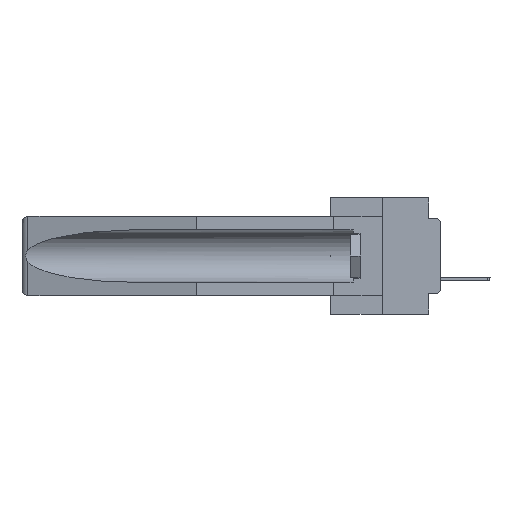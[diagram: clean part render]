
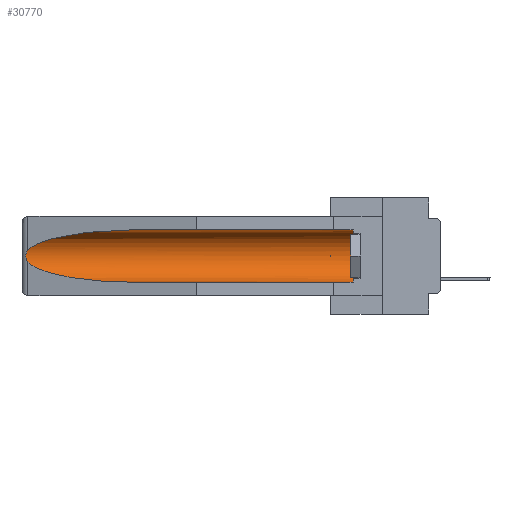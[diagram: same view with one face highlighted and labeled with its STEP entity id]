
A CAD part, left-side view. The second image highlights one B-rep face of the part: STEP entity #30770.
In plain terms, the highlighted cylindrical face has radius 2.857 mm (diameter 5.715 mm), a partial arc.
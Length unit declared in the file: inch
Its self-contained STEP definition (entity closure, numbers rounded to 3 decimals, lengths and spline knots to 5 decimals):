
#49 = CARTESIAN_POINT ( 'NONE',  ( 0.26537, 1.52718, -0.19328 ) ) ;
#94 = CARTESIAN_POINT ( 'NONE',  ( 0.155, 1.07973, -0.284 ) ) ;
#1596 = CARTESIAN_POINT ( 'NONE',  ( 0.26597, 1.52961, -0.15275 ) ) ;
#1840 = EDGE_LOOP ( 'NONE', ( #20788, #6467, #7239, #36404, #6667, #8755 ) ) ;
#1914 = CARTESIAN_POINT ( 'NONE',  ( 0.155, 0.126, -0.059 ) ) ;
#1947 =( BOUNDED_CURVE ( )  B_SPLINE_CURVE ( 3, ( #23305, #28876, #14259, #11176 ),
 .UNSPECIFIED., .F., .F. ) 
 B_SPLINE_CURVE_WITH_KNOTS ( ( 4, 4 ),
 ( 4.71239, 6.08839 ),
 .UNSPECIFIED. ) 
 CURVE ( )  GEOMETRIC_REPRESENTATION_ITEM ( )  RATIONAL_B_SPLINE_CURVE ( ( 1., 0.848, 0.848, 1. ) ) 
 REPRESENTATION_ITEM ( '' )  );
#1971 = EDGE_CURVE ( 'NONE', #37057, #34717, #27311, .T. ) ;
#2161 = AXIS2_PLACEMENT_3D ( 'NONE', #34331, #30947, #29024 ) ;
#4720 = CARTESIAN_POINT ( 'NONE',  ( 0.2675, 1.53308, -0.17534 ) ) ;
#4996 = CARTESIAN_POINT ( 'NONE',  ( 0.26537, 1.52718, -0.14972 ) ) ;
#5234 = CARTESIAN_POINT ( 'NONE',  ( 0.155, -0.30754, -0.1715 ) ) ;
#6221 = EDGE_CURVE ( 'NONE', #34717, #8247, #20496, .T. ) ;
#6467 = ORIENTED_EDGE ( 'NONE', *, *, #1971, .T. ) ;
#6667 = ORIENTED_EDGE ( 'NONE', *, *, #18655, .T. ) ;
#7239 = ORIENTED_EDGE ( 'NONE', *, *, #6221, .T. ) ;
#7348 = EDGE_CURVE ( 'NONE', #13202, #8247, #18905, .T. ) ;
#8247 = VERTEX_POINT ( 'NONE', #32689 ) ;
#8552 = CARTESIAN_POINT ( 'NONE',  ( 0.155, -0.30754, -0.059 ) ) ;
#8755 = ORIENTED_EDGE ( 'NONE', *, *, #23023, .T. ) ;
#9135 = CARTESIAN_POINT ( 'NONE',  ( 0.26537, 1.52718, -0.19328 ) ) ;
#10565 = CARTESIAN_POINT ( 'NONE',  ( 0.2673, 1.5327, -0.16383 ) ) ;
#11176 = CARTESIAN_POINT ( 'NONE',  ( 0.26537, 1.52718, -0.14972 ) ) ;
#11797 = DIRECTION ( 'NONE',  ( 0., 1., 0. ) ) ;
#13202 = VERTEX_POINT ( 'NONE', #31782 ) ;
#13942 = CARTESIAN_POINT ( 'NONE',  ( 0.26597, 1.5296, -0.19026 ) ) ;
#14259 = CARTESIAN_POINT ( 'NONE',  ( 0.25451, 1.48313, -0.09465 ) ) ;
#14314 = CARTESIAN_POINT ( 'NONE',  ( 0.26537, 1.52718, -0.19328 ) ) ;
#14658 = AXIS2_PLACEMENT_3D ( 'NONE', #5234, #28541, #28920 ) ;
#14791 = VECTOR ( 'NONE', #22043, 39.37008 ) ;
#15613 = CARTESIAN_POINT ( 'NONE',  ( 0.155, 1.07973, -0.059 ) ) ;
#16110 = CARTESIAN_POINT ( 'NONE',  ( 0.155, -0.30754, -0.284 ) ) ;
#16844 = CIRCLE ( 'NONE', #2161, 0.1125 ) ;
#17485 = VERTEX_POINT ( 'NONE', #15613 ) ;
#17597 = VECTOR ( 'NONE', #11797, 39.37008 ) ;
#18655 = EDGE_CURVE ( 'NONE', #13202, #33280, #16844, .T. ) ;
#18905 = LINE ( 'NONE', #16110, #14791 ) ;
#19532 = CARTESIAN_POINT ( 'NONE',  ( 0.26654, 1.53092, -0.15636 ) ) ;
#20056 = EDGE_CURVE ( 'NONE', #17485, #37057, #1947, .T. ) ;
#20496 =( BOUNDED_CURVE ( )  B_SPLINE_CURVE ( 3, ( #49, #20834, #21333, #94 ),
 .UNSPECIFIED., .F., .T. ) 
 B_SPLINE_CURVE_WITH_KNOTS ( ( 4, 4 ),
 ( 0.1948, 1.5708 ),
 .UNSPECIFIED. ) 
 CURVE ( )  GEOMETRIC_REPRESENTATION_ITEM ( )  RATIONAL_B_SPLINE_CURVE ( ( 1., 0.848, 0.848, 1. ) ) 
 REPRESENTATION_ITEM ( '' )  );
#20681 = CARTESIAN_POINT ( 'NONE',  ( 0.26537, 1.52718, -0.14972 ) ) ;
#20788 = ORIENTED_EDGE ( 'NONE', *, *, #20056, .T. ) ;
#20834 = CARTESIAN_POINT ( 'NONE',  ( 0.25451, 1.48313, -0.24835 ) ) ;
#21333 = CARTESIAN_POINT ( 'NONE',  ( 0.21114, 1.30732, -0.284 ) ) ;
#22043 = DIRECTION ( 'NONE',  ( 0., 1., 0. ) ) ;
#22226 = FACE_OUTER_BOUND ( 'NONE', #1840, .T. ) ;
#22462 = CARTESIAN_POINT ( 'NONE',  ( 0.2675, 1.53308, -0.16763 ) ) ;
#23023 = EDGE_CURVE ( 'NONE', #33280, #17485, #28685, .T. ) ;
#23305 = CARTESIAN_POINT ( 'NONE',  ( 0.155, 1.07973, -0.059 ) ) ;
#25476 = CARTESIAN_POINT ( 'NONE',  ( 0.2673, 1.53269, -0.17917 ) ) ;
#27311 = B_SPLINE_CURVE_WITH_KNOTS ( 'NONE', 3,
 ( #4996, #1596, #19532, #10565, #22462, #4720, #25476, #31799, #13942, #9135 ),
 .UNSPECIFIED., .F., .F.,
 ( 4, 2, 2, 2, 4 ),
 ( 0., 0.00029, 0.00058, 0.00087, 0.00117 ),
 .UNSPECIFIED. ) ;
#28541 = DIRECTION ( 'NONE',  ( 0., 1., 0. ) ) ;
#28685 = LINE ( 'NONE', #8552, #17597 ) ;
#28876 = CARTESIAN_POINT ( 'NONE',  ( 0.21114, 1.30732, -0.059 ) ) ;
#28920 = DIRECTION ( 'NONE',  ( 0., 0., 1. ) ) ;
#29024 = DIRECTION ( 'NONE',  ( 0., 0., 1. ) ) ;
#30770 = ADVANCED_FACE ( 'NONE', ( #22226 ), #37581, .F. ) ;
#30947 = DIRECTION ( 'NONE',  ( 0., -1., 0. ) ) ;
#31782 = CARTESIAN_POINT ( 'NONE',  ( 0.155, 0.126, -0.284 ) ) ;
#31799 = CARTESIAN_POINT ( 'NONE',  ( 0.26655, 1.53094, -0.18657 ) ) ;
#32689 = CARTESIAN_POINT ( 'NONE',  ( 0.155, 1.07973, -0.284 ) ) ;
#33280 = VERTEX_POINT ( 'NONE', #1914 ) ;
#34331 = CARTESIAN_POINT ( 'NONE',  ( 0.155, 0.126, -0.1715 ) ) ;
#34717 = VERTEX_POINT ( 'NONE', #14314 ) ;
#36404 = ORIENTED_EDGE ( 'NONE', *, *, #7348, .F. ) ;
#37057 = VERTEX_POINT ( 'NONE', #20681 ) ;
#37581 = CYLINDRICAL_SURFACE ( 'NONE', #14658, 0.1125 ) ;
